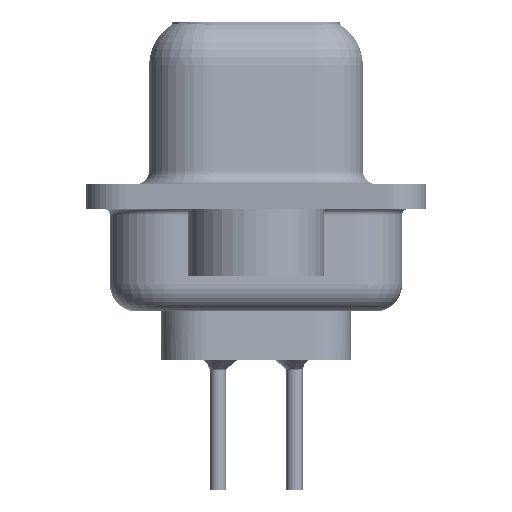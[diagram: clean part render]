
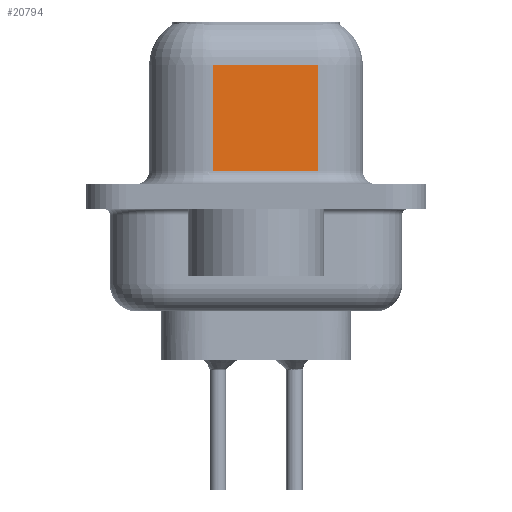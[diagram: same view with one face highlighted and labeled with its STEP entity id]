
A CAD part, left-side view. The second image highlights one B-rep face of the part: STEP entity #20794.
In plain terms, the highlighted planar face has unit normal (-0.985, -0.174, 0).
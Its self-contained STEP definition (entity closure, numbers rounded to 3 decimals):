
#136 = ORIENTED_EDGE ( 'NONE', *, *, #19158, .F. ) ;
#1076 = DIRECTION ( 'NONE',  ( 0.985, 0.174, 0. ) ) ;
#1263 = CARTESIAN_POINT ( 'NONE',  ( 4.38, 1.603, 0.95 ) ) ;
#2242 = LINE ( 'NONE', #17166, #4350 ) ;
#2947 = EDGE_CURVE ( 'NONE', #30627, #25812, #3566, .T. ) ;
#3245 = CARTESIAN_POINT ( 'NONE',  ( 5.068, -2.297, 6.6 ) ) ;
#3285 = VERTEX_POINT ( 'NONE', #23561 ) ;
#3566 = LINE ( 'NONE', #18647, #15711 ) ;
#4350 = VECTOR ( 'NONE', #20310, 1000. ) ;
#5706 = VERTEX_POINT ( 'NONE', #10863 ) ;
#6310 = EDGE_CURVE ( 'NONE', #25812, #3285, #32024, .T. ) ;
#6557 = AXIS2_PLACEMENT_3D ( 'NONE', #3245, #1076, #30751 ) ;
#8382 = FACE_OUTER_BOUND ( 'NONE', #25679, .T. ) ;
#8468 = LINE ( 'NONE', #28535, #26049 ) ;
#10863 = CARTESIAN_POINT ( 'NONE',  ( 5.068, -2.297, 4.85 ) ) ;
#15711 = VECTOR ( 'NONE', #29369, 1000. ) ;
#16599 = CARTESIAN_POINT ( 'NONE',  ( 5.068, -2.297, 0.95 ) ) ;
#16940 = DIRECTION ( 'NONE',  ( 0.174, -0.985, 0. ) ) ;
#17166 = CARTESIAN_POINT ( 'NONE',  ( 5.068, -2.297, 6.6 ) ) ;
#18647 = CARTESIAN_POINT ( 'NONE',  ( 4.38, 1.603, 6.6 ) ) ;
#19158 = EDGE_CURVE ( 'NONE', #5706, #3285, #2242, .T. ) ;
#19183 = ORIENTED_EDGE ( 'NONE', *, *, #6310, .T. ) ;
#20310 = DIRECTION ( 'NONE',  ( 0., 0., -1. ) ) ;
#20646 = PLANE ( 'NONE',  #6557 ) ;
#20794 = ADVANCED_FACE ( 'NONE', ( #8382 ), #20646, .F. ) ;
#23561 = CARTESIAN_POINT ( 'NONE',  ( 5.068, -2.297, 0.95 ) ) ;
#23728 = DIRECTION ( 'NONE',  ( -0.174, 0.985, 0. ) ) ;
#24391 = ORIENTED_EDGE ( 'NONE', *, *, #30285, .T. ) ;
#24981 = VECTOR ( 'NONE', #16940, 1000. ) ;
#25012 = CARTESIAN_POINT ( 'NONE',  ( 4.38, 1.603, 4.85 ) ) ;
#25679 = EDGE_LOOP ( 'NONE', ( #136, #24391, #30156, #19183 ) ) ;
#25812 = VERTEX_POINT ( 'NONE', #1263 ) ;
#26049 = VECTOR ( 'NONE', #23728, 1000. ) ;
#28535 = CARTESIAN_POINT ( 'NONE',  ( 5.068, -2.297, 4.85 ) ) ;
#29369 = DIRECTION ( 'NONE',  ( 0., 0., -1. ) ) ;
#30156 = ORIENTED_EDGE ( 'NONE', *, *, #2947, .T. ) ;
#30285 = EDGE_CURVE ( 'NONE', #5706, #30627, #8468, .T. ) ;
#30627 = VERTEX_POINT ( 'NONE', #25012 ) ;
#30751 = DIRECTION ( 'NONE',  ( -0.174, 0.985, 0. ) ) ;
#32024 = LINE ( 'NONE', #16599, #24981 ) ;
